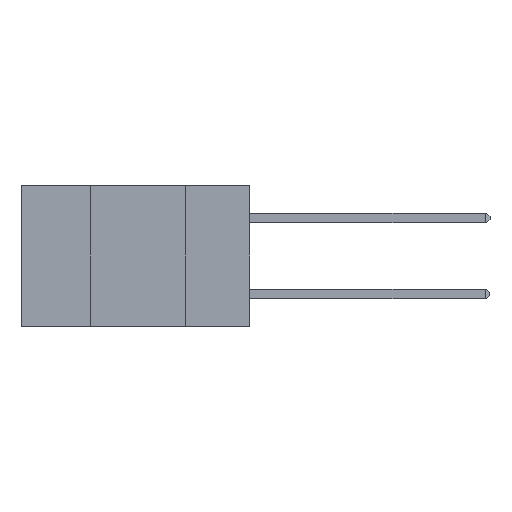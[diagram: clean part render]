
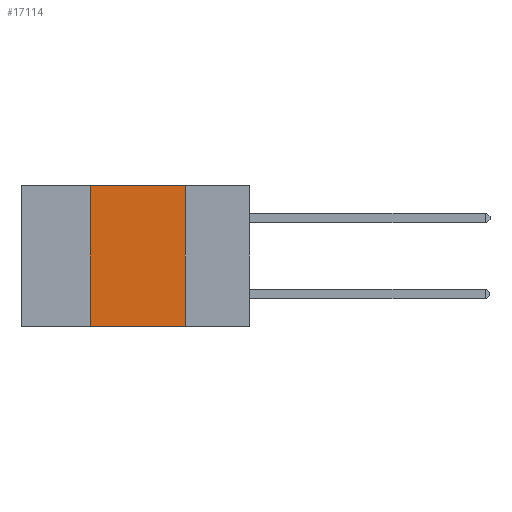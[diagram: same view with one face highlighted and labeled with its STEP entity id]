
A CAD part, left-side view. The second image highlights one B-rep face of the part: STEP entity #17114.
In plain terms, the highlighted planar face has unit normal (-1, 0, 0).
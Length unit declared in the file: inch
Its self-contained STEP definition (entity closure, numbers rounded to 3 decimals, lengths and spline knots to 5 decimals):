
#118 = VECTOR ( 'NONE', #5297, 39.37008 ) ;
#417 = CARTESIAN_POINT ( 'NONE',  ( 0., 0.17, 0. ) ) ;
#587 = FACE_OUTER_BOUND ( 'NONE', #9025, .T. ) ;
#734 = CARTESIAN_POINT ( 'NONE',  ( 0., 0.6, 0. ) ) ;
#812 = DIRECTION ( 'NONE',  ( 0., 0., -1. ) ) ;
#876 = CARTESIAN_POINT ( 'NONE',  ( 0., 0.17, 0. ) ) ;
#1474 = ORIENTED_EDGE ( 'NONE', *, *, #1957, .F. ) ;
#1957 = EDGE_CURVE ( 'NONE', #14872, #15616, #13511, .T. ) ;
#3153 = VERTEX_POINT ( 'NONE', #10915 ) ;
#3177 = VECTOR ( 'NONE', #16886, 39.37008 ) ;
#3233 = EDGE_CURVE ( 'NONE', #3153, #9011, #19779, .T. ) ;
#4262 = DIRECTION ( 'NONE',  ( 0., -1., 0. ) ) ;
#4922 = CARTESIAN_POINT ( 'NONE',  ( 0., 0.6, -0.37 ) ) ;
#5225 = CARTESIAN_POINT ( 'NONE',  ( 0., 0.17, -0.37 ) ) ;
#5297 = DIRECTION ( 'NONE',  ( 0., -1., 0. ) ) ;
#5494 = CARTESIAN_POINT ( 'NONE',  ( 0., 0.42, 0. ) ) ;
#7758 = EDGE_CURVE ( 'NONE', #3153, #14872, #19642, .T. ) ;
#8080 = AXIS2_PLACEMENT_3D ( 'NONE', #734, #10896, #812 ) ;
#9011 = VERTEX_POINT ( 'NONE', #5225 ) ;
#9025 = EDGE_LOOP ( 'NONE', ( #11704, #1474, #19817, #15008 ) ) ;
#9319 = EDGE_CURVE ( 'NONE', #15616, #9011, #10966, .T. ) ;
#10645 = VECTOR ( 'NONE', #4262, 39.37008 ) ;
#10896 = DIRECTION ( 'NONE',  ( 1., 0., 0. ) ) ;
#10915 = CARTESIAN_POINT ( 'NONE',  ( 0., 0.42, -0.37 ) ) ;
#10966 = LINE ( 'NONE', #876, #19134 ) ;
#11704 = ORIENTED_EDGE ( 'NONE', *, *, #9319, .F. ) ;
#13340 = CARTESIAN_POINT ( 'NONE',  ( 0., 0.6, 0. ) ) ;
#13511 = LINE ( 'NONE', #13340, #118 ) ;
#14872 = VERTEX_POINT ( 'NONE', #18250 ) ;
#15008 = ORIENTED_EDGE ( 'NONE', *, *, #3233, .T. ) ;
#15616 = VERTEX_POINT ( 'NONE', #417 ) ;
#15785 = DIRECTION ( 'NONE',  ( 0., 0., -1. ) ) ;
#16886 = DIRECTION ( 'NONE',  ( 0., 0., 1. ) ) ;
#17114 = ADVANCED_FACE ( 'NONE', ( #587 ), #20628, .F. ) ;
#18250 = CARTESIAN_POINT ( 'NONE',  ( 0., 0.42, 0. ) ) ;
#19134 = VECTOR ( 'NONE', #15785, 39.37008 ) ;
#19642 = LINE ( 'NONE', #5494, #3177 ) ;
#19779 = LINE ( 'NONE', #4922, #10645 ) ;
#19817 = ORIENTED_EDGE ( 'NONE', *, *, #7758, .F. ) ;
#20628 = PLANE ( 'NONE',  #8080 ) ;
